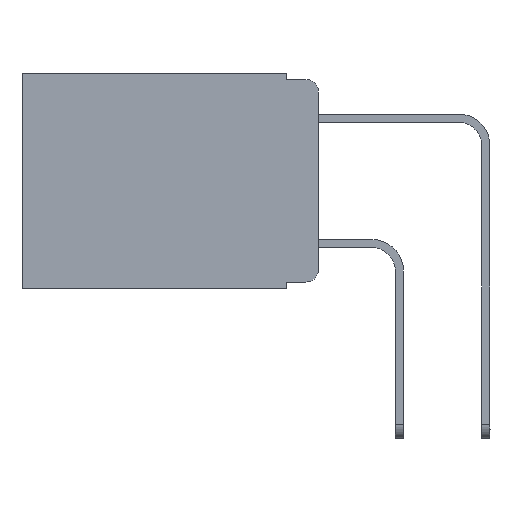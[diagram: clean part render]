
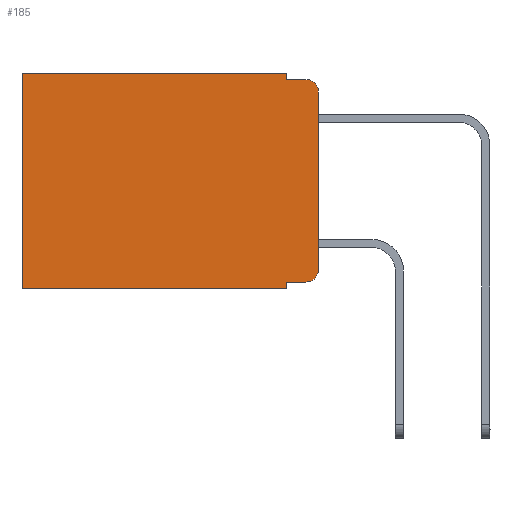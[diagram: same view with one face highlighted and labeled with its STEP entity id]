
A CAD part, left-side view. The second image highlights one B-rep face of the part: STEP entity #185.
In plain terms, the highlighted planar face has unit normal (-1, 0, 0).
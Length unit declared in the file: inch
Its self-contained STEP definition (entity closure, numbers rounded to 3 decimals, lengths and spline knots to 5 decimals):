
#185 = ADVANCED_FACE ( 'NONE', ( #1262 ), #5195, .F. ) ;
#207 = VERTEX_POINT ( 'NONE', #9779 ) ;
#608 = AXIS2_PLACEMENT_3D ( 'NONE', #7882, #9042, #12285 ) ;
#824 = LINE ( 'NONE', #6257, #7032 ) ;
#890 = LINE ( 'NONE', #4856, #10342 ) ;
#920 = CARTESIAN_POINT ( 'NONE',  ( 0.298, 0.473, -0.343 ) ) ;
#1060 = CARTESIAN_POINT ( 'NONE',  ( 0.298, 0., -0.313 ) ) ;
#1262 = FACE_OUTER_BOUND ( 'NONE', #4840, .T. ) ;
#1841 = ORIENTED_EDGE ( 'NONE', *, *, #11296, .T. ) ;
#2346 = VERTEX_POINT ( 'NONE', #2513 ) ;
#2434 = CIRCLE ( 'NONE', #14010, 0.02 ) ;
#2493 = EDGE_CURVE ( 'NONE', #11609, #7106, #824, .T. ) ;
#2513 = CARTESIAN_POINT ( 'NONE',  ( 0.298, 0.051, -0.01 ) ) ;
#2729 = CARTESIAN_POINT ( 'NONE',  ( 0.298, 0.02, -0.313 ) ) ;
#2895 = CARTESIAN_POINT ( 'NONE',  ( 0.298, 0., 0. ) ) ;
#2971 = VECTOR ( 'NONE', #12371, 39.37008 ) ;
#3479 = ORIENTED_EDGE ( 'NONE', *, *, #5676, .F. ) ;
#3954 = VECTOR ( 'NONE', #10441, 39.37008 ) ;
#3973 = ORIENTED_EDGE ( 'NONE', *, *, #5446, .T. ) ;
#4033 = ORIENTED_EDGE ( 'NONE', *, *, #9367, .F. ) ;
#4095 = AXIS2_PLACEMENT_3D ( 'NONE', #2895, #4202, #9682 ) ;
#4202 = DIRECTION ( 'NONE',  ( 1., 0., 0. ) ) ;
#4645 = CARTESIAN_POINT ( 'NONE',  ( 0.298, 0.051, -0.01 ) ) ;
#4655 = CARTESIAN_POINT ( 'NONE',  ( 0.298, 0., 0. ) ) ;
#4840 = EDGE_LOOP ( 'NONE', ( #10125, #7661, #4936, #4033, #11836, #1841, #3479, #6011, #3973, #5234 ) ) ;
#4856 = CARTESIAN_POINT ( 'NONE',  ( 0.298, 0.473, 0. ) ) ;
#4936 = ORIENTED_EDGE ( 'NONE', *, *, #10217, .F. ) ;
#5021 = EDGE_CURVE ( 'NONE', #13619, #14004, #12760, .T. ) ;
#5121 = DIRECTION ( 'NONE',  ( 0., 0., -1. ) ) ;
#5195 = PLANE ( 'NONE',  #4095 ) ;
#5234 = ORIENTED_EDGE ( 'NONE', *, *, #13632, .T. ) ;
#5363 = CARTESIAN_POINT ( 'NONE',  ( 0.298, 0.051, -0.333 ) ) ;
#5385 = LINE ( 'NONE', #4655, #3954 ) ;
#5446 = EDGE_CURVE ( 'NONE', #11609, #207, #12202, .T. ) ;
#5560 = VERTEX_POINT ( 'NONE', #11111 ) ;
#5676 = EDGE_CURVE ( 'NONE', #7106, #7097, #6778, .T. ) ;
#6011 = ORIENTED_EDGE ( 'NONE', *, *, #2493, .F. ) ;
#6074 = DIRECTION ( 'NONE',  ( 0., 0., -1. ) ) ;
#6077 = EDGE_CURVE ( 'NONE', #5560, #10554, #5385, .T. ) ;
#6119 = DIRECTION ( 'NONE',  ( 0., -1., 0. ) ) ;
#6257 = CARTESIAN_POINT ( 'NONE',  ( 0.298, 0.051, 0. ) ) ;
#6285 = VECTOR ( 'NONE', #7671, 39.37008 ) ;
#6432 = DIRECTION ( 'NONE',  ( 0., -1., 0. ) ) ;
#6491 = VECTOR ( 'NONE', #6119, 39.37008 ) ;
#6588 = VERTEX_POINT ( 'NONE', #1060 ) ;
#6778 = LINE ( 'NONE', #9353, #12747 ) ;
#6841 = LINE ( 'NONE', #4645, #6491 ) ;
#7032 = VECTOR ( 'NONE', #6074, 39.37008 ) ;
#7097 = VERTEX_POINT ( 'NONE', #920 ) ;
#7106 = VERTEX_POINT ( 'NONE', #7644 ) ;
#7644 = CARTESIAN_POINT ( 'NONE',  ( 0.298, 0.051, -0.343 ) ) ;
#7661 = ORIENTED_EDGE ( 'NONE', *, *, #5021, .T. ) ;
#7671 = DIRECTION ( 'NONE',  ( 0., 0., -1. ) ) ;
#7882 = CARTESIAN_POINT ( 'NONE',  ( 0.298, 0.02, -0.03 ) ) ;
#8378 = CARTESIAN_POINT ( 'NONE',  ( 0.298, 0., -0.03 ) ) ;
#8391 = VECTOR ( 'NONE', #6432, 39.37008 ) ;
#9042 = DIRECTION ( 'NONE',  ( -1., 0., 0. ) ) ;
#9137 = LINE ( 'NONE', #11073, #6285 ) ;
#9353 = CARTESIAN_POINT ( 'NONE',  ( 0.298, 0., -0.343 ) ) ;
#9367 = EDGE_CURVE ( 'NONE', #5560, #2346, #13711, .T. ) ;
#9682 = DIRECTION ( 'NONE',  ( 0., 0., -1. ) ) ;
#9699 = DIRECTION ( 'NONE',  ( -1., 0., 0. ) ) ;
#9779 = CARTESIAN_POINT ( 'NONE',  ( 0.298, 0.02, -0.333 ) ) ;
#9848 = DIRECTION ( 'NONE',  ( 0., 0., -1. ) ) ;
#10125 = ORIENTED_EDGE ( 'NONE', *, *, #14709, .F. ) ;
#10217 = EDGE_CURVE ( 'NONE', #2346, #14004, #6841, .T. ) ;
#10342 = VECTOR ( 'NONE', #9848, 39.37008 ) ;
#10441 = DIRECTION ( 'NONE',  ( 0., 1., 0. ) ) ;
#10554 = VERTEX_POINT ( 'NONE', #14604 ) ;
#11073 = CARTESIAN_POINT ( 'NONE',  ( 0.298, 0., 0. ) ) ;
#11111 = CARTESIAN_POINT ( 'NONE',  ( 0.298, 0.051, 0. ) ) ;
#11296 = EDGE_CURVE ( 'NONE', #10554, #7097, #890, .T. ) ;
#11307 = CARTESIAN_POINT ( 'NONE',  ( 0.298, 0.051, 0. ) ) ;
#11609 = VERTEX_POINT ( 'NONE', #13994 ) ;
#11836 = ORIENTED_EDGE ( 'NONE', *, *, #6077, .T. ) ;
#12202 = LINE ( 'NONE', #5363, #8391 ) ;
#12285 = DIRECTION ( 'NONE',  ( 0., 0., -1. ) ) ;
#12371 = DIRECTION ( 'NONE',  ( 0., 0., -1. ) ) ;
#12622 = CARTESIAN_POINT ( 'NONE',  ( 0.298, 0.02, -0.01 ) ) ;
#12747 = VECTOR ( 'NONE', #13996, 39.37008 ) ;
#12760 = CIRCLE ( 'NONE', #608, 0.02 ) ;
#13619 = VERTEX_POINT ( 'NONE', #8378 ) ;
#13632 = EDGE_CURVE ( 'NONE', #207, #6588, #2434, .T. ) ;
#13711 = LINE ( 'NONE', #11307, #2971 ) ;
#13994 = CARTESIAN_POINT ( 'NONE',  ( 0.298, 0.051, -0.333 ) ) ;
#13996 = DIRECTION ( 'NONE',  ( 0., 1., 0. ) ) ;
#14004 = VERTEX_POINT ( 'NONE', #12622 ) ;
#14010 = AXIS2_PLACEMENT_3D ( 'NONE', #2729, #9699, #5121 ) ;
#14604 = CARTESIAN_POINT ( 'NONE',  ( 0.298, 0.473, 0. ) ) ;
#14709 = EDGE_CURVE ( 'NONE', #13619, #6588, #9137, .T. ) ;
